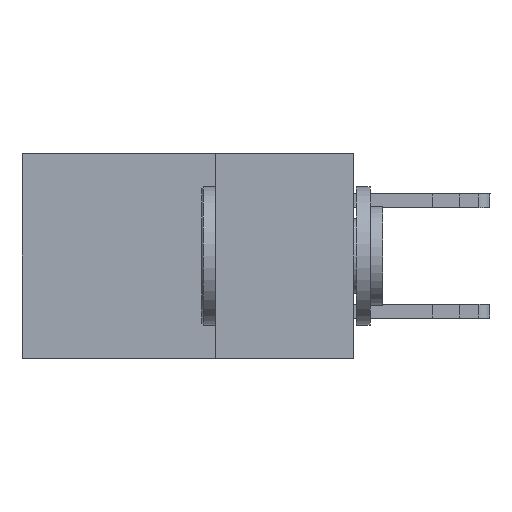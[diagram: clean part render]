
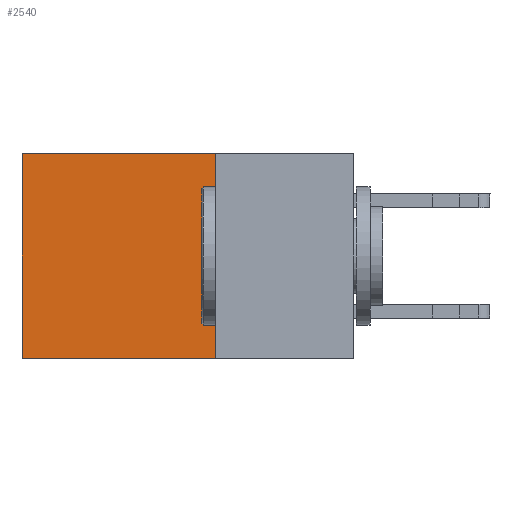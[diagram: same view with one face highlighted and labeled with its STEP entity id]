
A CAD part, left-side view. The second image highlights one B-rep face of the part: STEP entity #2540.
In plain terms, the highlighted planar face has unit normal (-1, 0, 0).
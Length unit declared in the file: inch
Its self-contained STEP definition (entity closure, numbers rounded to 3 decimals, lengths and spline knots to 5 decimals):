
#736 = DIRECTION ( 'NONE',  ( 1., 0., 0. ) ) ;
#1132 = CARTESIAN_POINT ( 'NONE',  ( 0.2875, 0.6, -0.37 ) ) ;
#1174 = EDGE_CURVE ( 'NONE', #21024, #24055, #16704, .T. ) ;
#1181 = VECTOR ( 'NONE', #6785, 39.37008 ) ;
#1569 = ORIENTED_EDGE ( 'NONE', *, *, #2938, .T. ) ;
#1843 = VERTEX_POINT ( 'NONE', #1132 ) ;
#2022 = AXIS2_PLACEMENT_3D ( 'NONE', #7475, #736, #11729 ) ;
#2268 = ORIENTED_EDGE ( 'NONE', *, *, #20362, .F. ) ;
#2540 = ADVANCED_FACE ( 'NONE', ( #21985 ), #9546, .F. ) ;
#2938 = EDGE_CURVE ( 'NONE', #24055, #1843, #15621, .T. ) ;
#2955 = CARTESIAN_POINT ( 'NONE',  ( 0.2875, 0.25, -0.37 ) ) ;
#3337 = LINE ( 'NONE', #14038, #22515 ) ;
#6436 = LINE ( 'NONE', #27081, #20444 ) ;
#6785 = DIRECTION ( 'NONE',  ( 0., 1., 0. ) ) ;
#7475 = CARTESIAN_POINT ( 'NONE',  ( 0.2875, 0.25, 0. ) ) ;
#7879 = DIRECTION ( 'NONE',  ( 0., 0., -1. ) ) ;
#9546 = PLANE ( 'NONE',  #2022 ) ;
#9570 = VERTEX_POINT ( 'NONE', #2955 ) ;
#9791 = DIRECTION ( 'NONE',  ( 0., 1., 0. ) ) ;
#11217 = VECTOR ( 'NONE', #19344, 39.37008 ) ;
#11729 = DIRECTION ( 'NONE',  ( 0., 0., -1. ) ) ;
#13076 = CARTESIAN_POINT ( 'NONE',  ( 0.2875, 0.6, 0. ) ) ;
#13604 = EDGE_LOOP ( 'NONE', ( #1569, #24700, #2268, #25630 ) ) ;
#14038 = CARTESIAN_POINT ( 'NONE',  ( 0.2875, 0.25, -0.37 ) ) ;
#14897 = CARTESIAN_POINT ( 'NONE',  ( 0.2875, 0.25, 0. ) ) ;
#15621 = LINE ( 'NONE', #13076, #11217 ) ;
#15780 = EDGE_CURVE ( 'NONE', #9570, #1843, #3337, .T. ) ;
#16704 = LINE ( 'NONE', #19685, #1181 ) ;
#19344 = DIRECTION ( 'NONE',  ( 0., 0., -1. ) ) ;
#19685 = CARTESIAN_POINT ( 'NONE',  ( 0.2875, 0.25, 0. ) ) ;
#20362 = EDGE_CURVE ( 'NONE', #21024, #9570, #6436, .T. ) ;
#20444 = VECTOR ( 'NONE', #7879, 39.37008 ) ;
#21024 = VERTEX_POINT ( 'NONE', #14897 ) ;
#21985 = FACE_OUTER_BOUND ( 'NONE', #13604, .T. ) ;
#22515 = VECTOR ( 'NONE', #9791, 39.37008 ) ;
#24055 = VERTEX_POINT ( 'NONE', #25907 ) ;
#24700 = ORIENTED_EDGE ( 'NONE', *, *, #15780, .F. ) ;
#25630 = ORIENTED_EDGE ( 'NONE', *, *, #1174, .T. ) ;
#25907 = CARTESIAN_POINT ( 'NONE',  ( 0.2875, 0.6, 0. ) ) ;
#27081 = CARTESIAN_POINT ( 'NONE',  ( 0.2875, 0.25, 0. ) ) ;
